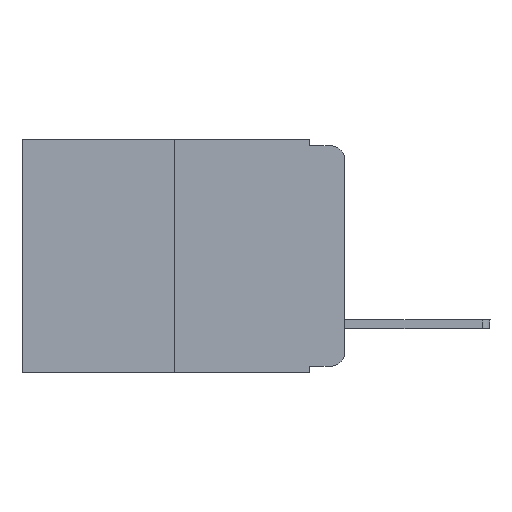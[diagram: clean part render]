
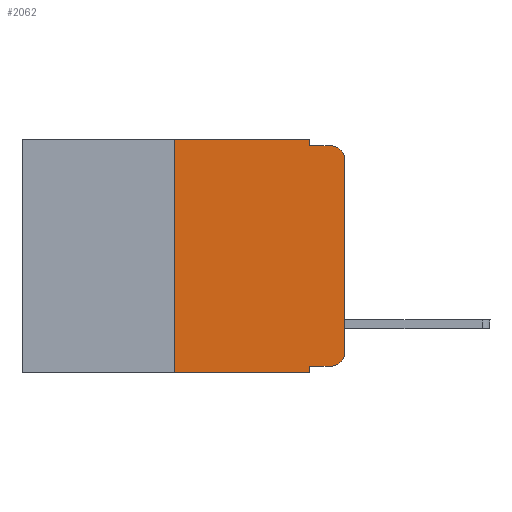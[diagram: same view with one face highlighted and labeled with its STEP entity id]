
A CAD part, left-side view. The second image highlights one B-rep face of the part: STEP entity #2062.
In plain terms, the highlighted planar face has unit normal (-1, 0, 0).
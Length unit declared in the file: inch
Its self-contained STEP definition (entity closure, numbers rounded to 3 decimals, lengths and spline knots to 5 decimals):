
#351 = VERTEX_POINT ( 'NONE', #20227 ) ;
#782 = DIRECTION ( 'NONE',  ( 0., 0., -1. ) ) ;
#790 = VERTEX_POINT ( 'NONE', #16487 ) ;
#956 = VERTEX_POINT ( 'NONE', #9907 ) ;
#1603 = ORIENTED_EDGE ( 'NONE', *, *, #18482, .F. ) ;
#2062 = ADVANCED_FACE ( 'NONE', ( #10348 ), #3582, .F. ) ;
#2325 = VECTOR ( 'NONE', #10994, 39.37008 ) ;
#2526 = CARTESIAN_POINT ( 'NONE',  ( 0., 0.051, 0. ) ) ;
#2527 = EDGE_CURVE ( 'NONE', #790, #14198, #16216, .T. ) ;
#2913 = VECTOR ( 'NONE', #21284, 39.37008 ) ;
#3122 = LINE ( 'NONE', #16382, #19055 ) ;
#3385 = CARTESIAN_POINT ( 'NONE',  ( 0., 0.473, 0. ) ) ;
#3466 = ORIENTED_EDGE ( 'NONE', *, *, #9240, .F. ) ;
#3582 = PLANE ( 'NONE',  #10086 ) ;
#3841 = CARTESIAN_POINT ( 'NONE',  ( 0., 0.051, 0. ) ) ;
#4231 = DIRECTION ( 'NONE',  ( -1., 0., 0. ) ) ;
#4380 = VERTEX_POINT ( 'NONE', #13543 ) ;
#4452 = EDGE_CURVE ( 'NONE', #4764, #12568, #11082, .T. ) ;
#4543 = EDGE_CURVE ( 'NONE', #6261, #4380, #10001, .T. ) ;
#4764 = VERTEX_POINT ( 'NONE', #17482 ) ;
#4949 = VECTOR ( 'NONE', #12737, 39.37008 ) ;
#5036 = LINE ( 'NONE', #17788, #2913 ) ;
#5197 = DIRECTION ( 'NONE',  ( 1., 0., 0. ) ) ;
#5694 = CARTESIAN_POINT ( 'NONE',  ( 0., 0.473, -0.343 ) ) ;
#5759 = CARTESIAN_POINT ( 'NONE',  ( 0., 0.051, -0.333 ) ) ;
#5926 = DIRECTION ( 'NONE',  ( 0., 0., -1. ) ) ;
#6261 = VERTEX_POINT ( 'NONE', #8429 ) ;
#6281 = ORIENTED_EDGE ( 'NONE', *, *, #2527, .F. ) ;
#6544 = VERTEX_POINT ( 'NONE', #19916 ) ;
#7013 = AXIS2_PLACEMENT_3D ( 'NONE', #11521, #11670, #13144 ) ;
#7322 = ORIENTED_EDGE ( 'NONE', *, *, #13087, .T. ) ;
#8429 = CARTESIAN_POINT ( 'NONE',  ( 0., 0., -0.313 ) ) ;
#8463 = VECTOR ( 'NONE', #13778, 39.37008 ) ;
#9240 = EDGE_CURVE ( 'NONE', #14198, #351, #21859, .T. ) ;
#9437 = DIRECTION ( 'NONE',  ( 0., -1., 0. ) ) ;
#9850 = EDGE_LOOP ( 'NONE', ( #17081, #11189, #18365, #3466, #6281, #1603, #12456, #13348, #7322, #20218 ) ) ;
#9907 = CARTESIAN_POINT ( 'NONE',  ( 0., 0.02, -0.333 ) ) ;
#10001 = LINE ( 'NONE', #15296, #13469 ) ;
#10086 = AXIS2_PLACEMENT_3D ( 'NONE', #12195, #5197, #17171 ) ;
#10348 = FACE_OUTER_BOUND ( 'NONE', #9850, .T. ) ;
#10994 = DIRECTION ( 'NONE',  ( 0., -1., 0. ) ) ;
#11082 = LINE ( 'NONE', #5694, #4949 ) ;
#11086 = CARTESIAN_POINT ( 'NONE',  ( 0., 0.051, -0.343 ) ) ;
#11189 = ORIENTED_EDGE ( 'NONE', *, *, #12512, .T. ) ;
#11438 = LINE ( 'NONE', #5759, #2325 ) ;
#11521 = CARTESIAN_POINT ( 'NONE',  ( 0., 0.02, -0.313 ) ) ;
#11670 = DIRECTION ( 'NONE',  ( -1., 0., 0. ) ) ;
#11892 = CIRCLE ( 'NONE', #18495, 0.02 ) ;
#12195 = CARTESIAN_POINT ( 'NONE',  ( 0., 0.473, 0. ) ) ;
#12456 = ORIENTED_EDGE ( 'NONE', *, *, #4452, .T. ) ;
#12512 = EDGE_CURVE ( 'NONE', #4380, #6544, #11892, .T. ) ;
#12546 = EDGE_CURVE ( 'NONE', #351, #6544, #3122, .T. ) ;
#12568 = VERTEX_POINT ( 'NONE', #11086 ) ;
#12737 = DIRECTION ( 'NONE',  ( 0., -1., 0. ) ) ;
#13087 = EDGE_CURVE ( 'NONE', #19655, #956, #11438, .T. ) ;
#13144 = DIRECTION ( 'NONE',  ( 0., 0., -1. ) ) ;
#13348 = ORIENTED_EDGE ( 'NONE', *, *, #18410, .F. ) ;
#13469 = VECTOR ( 'NONE', #17050, 39.37008 ) ;
#13543 = CARTESIAN_POINT ( 'NONE',  ( 0., 0., -0.03 ) ) ;
#13778 = DIRECTION ( 'NONE',  ( 0., -1., 0. ) ) ;
#14198 = VERTEX_POINT ( 'NONE', #2526 ) ;
#14433 = CARTESIAN_POINT ( 'NONE',  ( 0., 0.02, -0.03 ) ) ;
#14577 = CARTESIAN_POINT ( 'NONE',  ( 0., 0.051, -0.333 ) ) ;
#15296 = CARTESIAN_POINT ( 'NONE',  ( 0., 0., 0. ) ) ;
#15313 = EDGE_CURVE ( 'NONE', #956, #6261, #19771, .T. ) ;
#15972 = VECTOR ( 'NONE', #17444, 39.37008 ) ;
#16216 = LINE ( 'NONE', #3385, #8463 ) ;
#16239 = CARTESIAN_POINT ( 'NONE',  ( 0., 0.051, 0. ) ) ;
#16382 = CARTESIAN_POINT ( 'NONE',  ( 0., 0.051, -0.01 ) ) ;
#16487 = CARTESIAN_POINT ( 'NONE',  ( 0., 0.25, 0. ) ) ;
#17050 = DIRECTION ( 'NONE',  ( 0., 0., 1. ) ) ;
#17081 = ORIENTED_EDGE ( 'NONE', *, *, #4543, .T. ) ;
#17171 = DIRECTION ( 'NONE',  ( 0., 0., -1. ) ) ;
#17444 = DIRECTION ( 'NONE',  ( 0., 0., -1. ) ) ;
#17482 = CARTESIAN_POINT ( 'NONE',  ( 0., 0.25, -0.343 ) ) ;
#17788 = CARTESIAN_POINT ( 'NONE',  ( 0., 0.25, 0. ) ) ;
#18365 = ORIENTED_EDGE ( 'NONE', *, *, #12546, .F. ) ;
#18410 = EDGE_CURVE ( 'NONE', #19655, #12568, #21511, .T. ) ;
#18482 = EDGE_CURVE ( 'NONE', #4764, #790, #5036, .T. ) ;
#18495 = AXIS2_PLACEMENT_3D ( 'NONE', #14433, #4231, #5926 ) ;
#19055 = VECTOR ( 'NONE', #9437, 39.37008 ) ;
#19655 = VERTEX_POINT ( 'NONE', #14577 ) ;
#19688 = VECTOR ( 'NONE', #782, 39.37008 ) ;
#19771 = CIRCLE ( 'NONE', #7013, 0.02 ) ;
#19916 = CARTESIAN_POINT ( 'NONE',  ( 0., 0.02, -0.01 ) ) ;
#20218 = ORIENTED_EDGE ( 'NONE', *, *, #15313, .T. ) ;
#20227 = CARTESIAN_POINT ( 'NONE',  ( 0., 0.051, -0.01 ) ) ;
#21284 = DIRECTION ( 'NONE',  ( 0., 0., 1. ) ) ;
#21511 = LINE ( 'NONE', #3841, #15972 ) ;
#21859 = LINE ( 'NONE', #16239, #19688 ) ;
